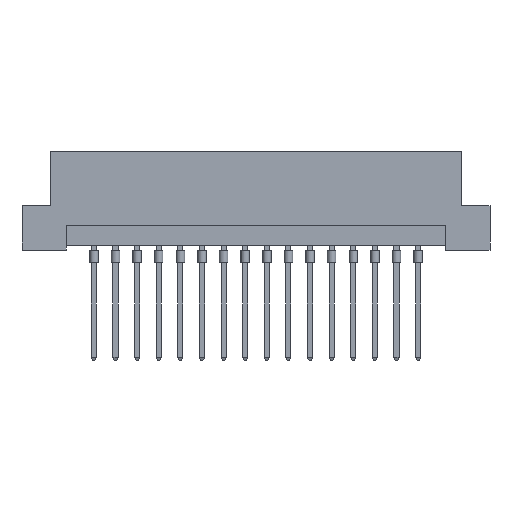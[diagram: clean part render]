
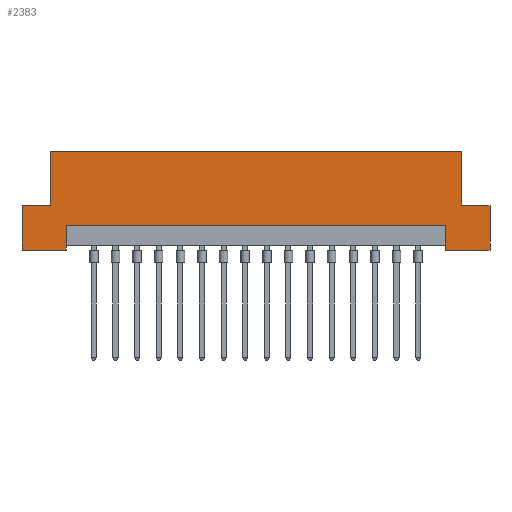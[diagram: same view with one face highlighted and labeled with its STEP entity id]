
A CAD part, front view. The second image highlights one B-rep face of the part: STEP entity #2383.
In plain terms, the highlighted planar face has unit normal (0, -1, 0).
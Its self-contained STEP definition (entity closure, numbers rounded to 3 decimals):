
#40 = VERTEX_POINT ( 'NONE', #9533 ) ;
#77 = LINE ( 'NONE', #6016, #2876 ) ;
#84 = ORIENTED_EDGE ( 'NONE', *, *, #5209, .F. ) ;
#98 = EDGE_CURVE ( 'NONE', #4126, #5750, #605, .T. ) ;
#273 = VECTOR ( 'NONE', #7831, 1000. ) ;
#295 = VERTEX_POINT ( 'NONE', #8230 ) ;
#373 = LINE ( 'NONE', #3301, #1886 ) ;
#426 = DIRECTION ( 'NONE',  ( -1., 0., 0. ) ) ;
#445 = DIRECTION ( 'NONE',  ( 1., 0., 0. ) ) ;
#512 = CARTESIAN_POINT ( 'NONE',  ( -22.3, 0., 0.5 ) ) ;
#605 = LINE ( 'NONE', #9440, #5129 ) ;
#722 = CARTESIAN_POINT ( 'NONE',  ( 22.3, 0., 2.9 ) ) ;
#765 = EDGE_CURVE ( 'NONE', #8555, #4996, #373, .T. ) ;
#920 = DIRECTION ( 'NONE',  ( 1., 0., 0. ) ) ;
#954 = VERTEX_POINT ( 'NONE', #5350 ) ;
#1018 = VECTOR ( 'NONE', #920, 1000. ) ;
#1133 = CARTESIAN_POINT ( 'NONE',  ( 27.5, 0., 5.2 ) ) ;
#1144 = LINE ( 'NONE', #4065, #9521 ) ;
#1369 = VERTEX_POINT ( 'NONE', #5794 ) ;
#1433 = FACE_OUTER_BOUND ( 'NONE', #4064, .T. ) ;
#1448 = EDGE_CURVE ( 'NONE', #5750, #954, #3768, .T. ) ;
#1767 = ORIENTED_EDGE ( 'NONE', *, *, #7782, .F. ) ;
#1812 = VECTOR ( 'NONE', #445, 1000. ) ;
#1846 = ORIENTED_EDGE ( 'NONE', *, *, #6852, .T. ) ;
#1886 = VECTOR ( 'NONE', #5040, 1000. ) ;
#1918 = VERTEX_POINT ( 'NONE', #2938 ) ;
#2330 = ORIENTED_EDGE ( 'NONE', *, *, #6693, .F. ) ;
#2383 = ADVANCED_FACE ( 'NONE', ( #1433 ), #7295, .F. ) ;
#2424 = DIRECTION ( 'NONE',  ( 0., 0., -1. ) ) ;
#2642 = VERTEX_POINT ( 'NONE', #4016 ) ;
#2649 = CARTESIAN_POINT ( 'NONE',  ( -27.5, 0., 5.2 ) ) ;
#2669 = ORIENTED_EDGE ( 'NONE', *, *, #765, .F. ) ;
#2876 = VECTOR ( 'NONE', #2424, 1000. ) ;
#2938 = CARTESIAN_POINT ( 'NONE',  ( -27.5, 0., 5.2 ) ) ;
#2971 = ORIENTED_EDGE ( 'NONE', *, *, #8049, .F. ) ;
#3188 = CARTESIAN_POINT ( 'NONE',  ( -27.5, 0., 0. ) ) ;
#3194 = VECTOR ( 'NONE', #9199, 1000. ) ;
#3301 = CARTESIAN_POINT ( 'NONE',  ( 22.3, 0., 2.9 ) ) ;
#3327 = LINE ( 'NONE', #4784, #3194 ) ;
#3570 = CARTESIAN_POINT ( 'NONE',  ( -27.5, 0., 11.6 ) ) ;
#3603 = CARTESIAN_POINT ( 'NONE',  ( -27.5, 0., 0. ) ) ;
#3720 = EDGE_CURVE ( 'NONE', #295, #4416, #1144, .T. ) ;
#3763 = DIRECTION ( 'NONE',  ( 0., 0., -1. ) ) ;
#3768 = LINE ( 'NONE', #3570, #7005 ) ;
#4016 = CARTESIAN_POINT ( 'NONE',  ( 27.5, 0., 0. ) ) ;
#4064 = EDGE_LOOP ( 'NONE', ( #2669, #1846, #6346, #1767, #84, #5435, #5966, #4790, #2971, #9349, #6459, #2330 ) ) ;
#4065 = CARTESIAN_POINT ( 'NONE',  ( -27.5, 0., 0. ) ) ;
#4126 = VERTEX_POINT ( 'NONE', #4650 ) ;
#4316 = CARTESIAN_POINT ( 'NONE',  ( -22.3, 0., 2.9 ) ) ;
#4416 = VERTEX_POINT ( 'NONE', #8081 ) ;
#4561 = LINE ( 'NONE', #4612, #1018 ) ;
#4612 = CARTESIAN_POINT ( 'NONE',  ( 27.5, 0., 5.2 ) ) ;
#4650 = CARTESIAN_POINT ( 'NONE',  ( -24.2, 0., 5.2 ) ) ;
#4743 = VECTOR ( 'NONE', #6619, 1000. ) ;
#4784 = CARTESIAN_POINT ( 'NONE',  ( 24.2, 0., 5.2 ) ) ;
#4790 = ORIENTED_EDGE ( 'NONE', *, *, #98, .F. ) ;
#4996 = VERTEX_POINT ( 'NONE', #4316 ) ;
#5040 = DIRECTION ( 'NONE',  ( -1., 0., 0. ) ) ;
#5129 = VECTOR ( 'NONE', #6583, 1000. ) ;
#5209 = EDGE_CURVE ( 'NONE', #1369, #6628, #4561, .T. ) ;
#5264 = CARTESIAN_POINT ( 'NONE',  ( 27.5, 0., 0. ) ) ;
#5350 = CARTESIAN_POINT ( 'NONE',  ( 24.2, 0., 11.6 ) ) ;
#5435 = ORIENTED_EDGE ( 'NONE', *, *, #7506, .T. ) ;
#5750 = VERTEX_POINT ( 'NONE', #9198 ) ;
#5794 = CARTESIAN_POINT ( 'NONE',  ( 24.2, 0., 5.2 ) ) ;
#5966 = ORIENTED_EDGE ( 'NONE', *, *, #1448, .F. ) ;
#6016 = CARTESIAN_POINT ( 'NONE',  ( 22.3, 0., 0.5 ) ) ;
#6286 = VECTOR ( 'NONE', #6947, 1000. ) ;
#6346 = ORIENTED_EDGE ( 'NONE', *, *, #8136, .F. ) ;
#6459 = ORIENTED_EDGE ( 'NONE', *, *, #3720, .F. ) ;
#6583 = DIRECTION ( 'NONE',  ( 0., 0., 1. ) ) ;
#6619 = DIRECTION ( 'NONE',  ( -1., 0., 0. ) ) ;
#6628 = VERTEX_POINT ( 'NONE', #1133 ) ;
#6693 = EDGE_CURVE ( 'NONE', #4996, #295, #9308, .T. ) ;
#6771 = LINE ( 'NONE', #3603, #4743 ) ;
#6852 = EDGE_CURVE ( 'NONE', #8555, #40, #77, .T. ) ;
#6947 = DIRECTION ( 'NONE',  ( 0., 0., -1. ) ) ;
#6985 = EDGE_CURVE ( 'NONE', #4416, #1918, #8569, .T. ) ;
#7005 = VECTOR ( 'NONE', #7316, 1000. ) ;
#7199 = DIRECTION ( 'NONE',  ( 0., 1., 0. ) ) ;
#7295 = PLANE ( 'NONE',  #9173 ) ;
#7316 = DIRECTION ( 'NONE',  ( 1., 0., 0. ) ) ;
#7355 = LINE ( 'NONE', #5264, #8307 ) ;
#7506 = EDGE_CURVE ( 'NONE', #1369, #954, #3327, .T. ) ;
#7782 = EDGE_CURVE ( 'NONE', #6628, #2642, #7355, .T. ) ;
#7831 = DIRECTION ( 'NONE',  ( 0., 0., 1. ) ) ;
#7908 = DIRECTION ( 'NONE',  ( 0., 0., 1. ) ) ;
#7913 = LINE ( 'NONE', #2649, #1812 ) ;
#8049 = EDGE_CURVE ( 'NONE', #1918, #4126, #7913, .T. ) ;
#8081 = CARTESIAN_POINT ( 'NONE',  ( -27.5, 0., 0. ) ) ;
#8136 = EDGE_CURVE ( 'NONE', #2642, #40, #6771, .T. ) ;
#8230 = CARTESIAN_POINT ( 'NONE',  ( -22.3, 0., 0. ) ) ;
#8307 = VECTOR ( 'NONE', #3763, 1000. ) ;
#8555 = VERTEX_POINT ( 'NONE', #722 ) ;
#8569 = LINE ( 'NONE', #3188, #273 ) ;
#9173 = AXIS2_PLACEMENT_3D ( 'NONE', #9466, #7199, #7908 ) ;
#9198 = CARTESIAN_POINT ( 'NONE',  ( -24.2, 0., 11.6 ) ) ;
#9199 = DIRECTION ( 'NONE',  ( 0., 0., 1. ) ) ;
#9308 = LINE ( 'NONE', #512, #6286 ) ;
#9349 = ORIENTED_EDGE ( 'NONE', *, *, #6985, .F. ) ;
#9440 = CARTESIAN_POINT ( 'NONE',  ( -24.2, 0., 5.2 ) ) ;
#9466 = CARTESIAN_POINT ( 'NONE',  ( -27.5, 0., 11.6 ) ) ;
#9521 = VECTOR ( 'NONE', #426, 1000. ) ;
#9533 = CARTESIAN_POINT ( 'NONE',  ( 22.3, 0., 0. ) ) ;
